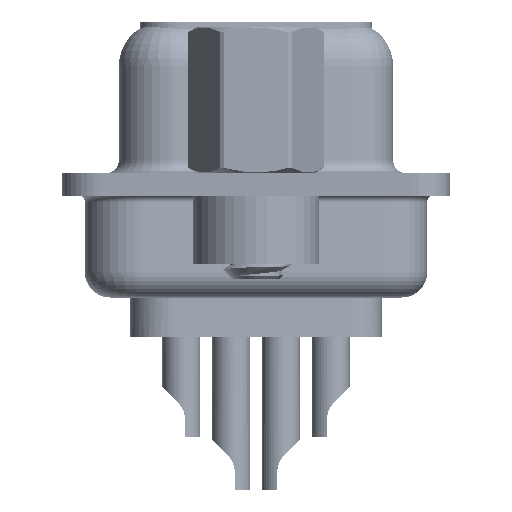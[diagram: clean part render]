
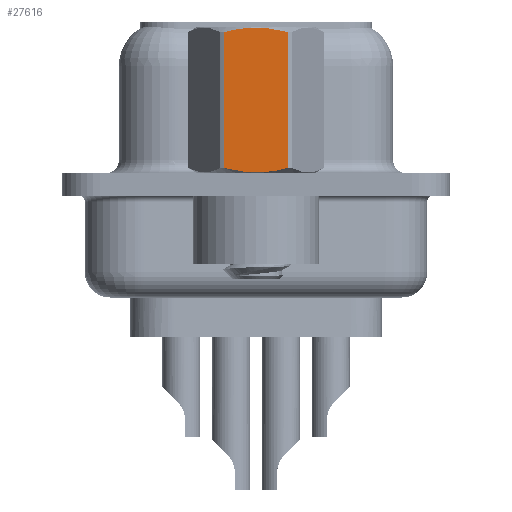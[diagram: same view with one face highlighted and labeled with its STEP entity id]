
A CAD part, left-side view. The second image highlights one B-rep face of the part: STEP entity #27616.
In plain terms, the highlighted planar face has unit normal (-1, 0, 0).
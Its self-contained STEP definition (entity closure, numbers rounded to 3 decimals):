
#3160 = CARTESIAN_POINT ( 'NONE',  ( -2.381, -0.858, 6.15 ) ) ;
#3611 = VECTOR ( 'NONE', #41808, 1000. ) ;
#5049 = CARTESIAN_POINT ( 'NONE',  ( -2.381, -1.273, 0.652 ) ) ;
#6929 = ORIENTED_EDGE ( 'NONE', *, *, #26958, .T. ) ;
#7519 = CARTESIAN_POINT ( 'NONE',  ( -2.381, 0.215, 6.232 ) ) ;
#7809 = CARTESIAN_POINT ( 'NONE',  ( -2.381, -0.215, 6.232 ) ) ;
#8094 = CARTESIAN_POINT ( 'NONE',  ( -2.381, -1.066, 6.104 ) ) ;
#8223 = VECTOR ( 'NONE', #45205, 1000. ) ;
#8679 = VERTEX_POINT ( 'NONE', #5049 ) ;
#11398 = CARTESIAN_POINT ( 'NONE',  ( -2.381, -0.432, 0.485 ) ) ;
#11690 = CARTESIAN_POINT ( 'NONE',  ( -2.381, 0.215, 0.468 ) ) ;
#12664 = AXIS2_PLACEMENT_3D ( 'NONE', #55973, #15472, #37930 ) ;
#13306 = ORIENTED_EDGE ( 'NONE', *, *, #30017, .T. ) ;
#14037 = CARTESIAN_POINT ( 'NONE',  ( -2.381, 1.273, 3.792 ) ) ;
#15472 = DIRECTION ( 'NONE',  ( -1., 0., 0. ) ) ;
#17143 = CARTESIAN_POINT ( 'NONE',  ( -2.381, -1.273, 6.048 ) ) ;
#20712 = FACE_OUTER_BOUND ( 'NONE', #46492, .T. ) ;
#22871 = VERTEX_POINT ( 'NONE', #30633 ) ;
#25117 = CARTESIAN_POINT ( 'NONE',  ( -2.381, -0.215, 0.468 ) ) ;
#25474 = B_SPLINE_CURVE_WITH_KNOTS ( 'NONE', 3,
 ( #17143, #8094, #3160, #25897, #7809, #7519, #48586, #39297, #56769, #30280 ),
 .UNSPECIFIED., .F., .F.,
 ( 4, 2, 2, 2, 4 ),
 ( 0.001, 0.002, 0.002, 0.003, 0.004 ),
 .UNSPECIFIED. ) ;
#25897 = CARTESIAN_POINT ( 'NONE',  ( -2.381, -0.432, 6.215 ) ) ;
#26958 = EDGE_CURVE ( 'NONE', #8679, #39851, #50817, .T. ) ;
#27616 = ADVANCED_FACE ( 'NONE', ( #20712 ), #33845, .T. ) ;
#29187 = CARTESIAN_POINT ( 'NONE',  ( -2.381, -1.273, 0.652 ) ) ;
#29759 = CARTESIAN_POINT ( 'NONE',  ( -2.381, 1.273, 0.652 ) ) ;
#30017 = EDGE_CURVE ( 'NONE', #46500, #8679, #46414, .T. ) ;
#30280 = CARTESIAN_POINT ( 'NONE',  ( -2.381, 1.273, 6.048 ) ) ;
#30585 = EDGE_CURVE ( 'NONE', #39851, #22871, #25474, .T. ) ;
#30633 = CARTESIAN_POINT ( 'NONE',  ( -2.381, 1.273, 6.048 ) ) ;
#31531 = LINE ( 'NONE', #14037, #8223 ) ;
#33845 = PLANE ( 'NONE',  #12664 ) ;
#36669 = ORIENTED_EDGE ( 'NONE', *, *, #30585, .T. ) ;
#37884 = CARTESIAN_POINT ( 'NONE',  ( -2.381, 1.273, 0.652 ) ) ;
#37930 = DIRECTION ( 'NONE',  ( 0., -1., 0. ) ) ;
#38230 = CARTESIAN_POINT ( 'NONE',  ( -2.381, 0.853, 0.549 ) ) ;
#39297 = CARTESIAN_POINT ( 'NONE',  ( -2.381, 0.853, 6.151 ) ) ;
#39851 = VERTEX_POINT ( 'NONE', #48550 ) ;
#41515 = CARTESIAN_POINT ( 'NONE',  ( -2.381, -1.066, 0.596 ) ) ;
#41808 = DIRECTION ( 'NONE',  ( 0., 0., 1. ) ) ;
#42881 = CARTESIAN_POINT ( 'NONE',  ( -2.381, -0.858, 0.55 ) ) ;
#43629 = EDGE_CURVE ( 'NONE', #22871, #46500, #31531, .T. ) ;
#45205 = DIRECTION ( 'NONE',  ( 0., 0., -1. ) ) ;
#46414 = B_SPLINE_CURVE_WITH_KNOTS ( 'NONE', 3,
 ( #29759, #51617, #38230, #55687, #11690, #25117, #11398, #42881, #41515, #29187 ),
 .UNSPECIFIED., .F., .F.,
 ( 4, 2, 2, 2, 4 ),
 ( 0.003, 0.003, 0.004, 0.004, 0.005 ),
 .UNSPECIFIED. ) ;
#46492 = EDGE_LOOP ( 'NONE', ( #13306, #6929, #36669, #55985 ) ) ;
#46500 = VERTEX_POINT ( 'NONE', #37884 ) ;
#48550 = CARTESIAN_POINT ( 'NONE',  ( -2.381, -1.273, 6.048 ) ) ;
#48586 = CARTESIAN_POINT ( 'NONE',  ( -2.381, 0.428, 6.215 ) ) ;
#50817 = LINE ( 'NONE', #54321, #3611 ) ;
#51617 = CARTESIAN_POINT ( 'NONE',  ( -2.381, 1.065, 0.596 ) ) ;
#54321 = CARTESIAN_POINT ( 'NONE',  ( -2.381, -1.273, 3.792 ) ) ;
#55687 = CARTESIAN_POINT ( 'NONE',  ( -2.381, 0.428, 0.485 ) ) ;
#55973 = CARTESIAN_POINT ( 'NONE',  ( -2.381, 1.375, -3.75 ) ) ;
#55985 = ORIENTED_EDGE ( 'NONE', *, *, #43629, .T. ) ;
#56769 = CARTESIAN_POINT ( 'NONE',  ( -2.381, 1.065, 6.104 ) ) ;
